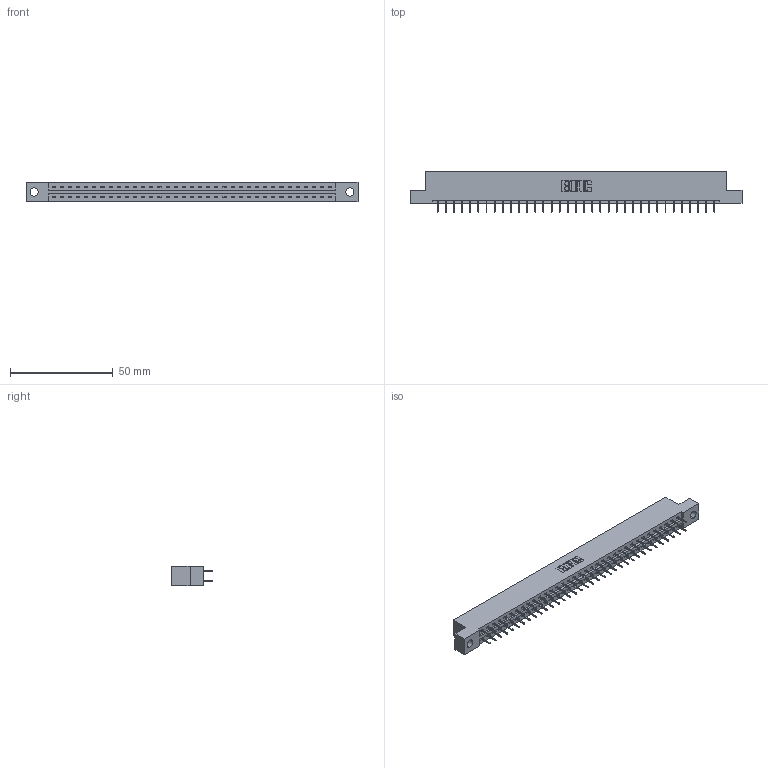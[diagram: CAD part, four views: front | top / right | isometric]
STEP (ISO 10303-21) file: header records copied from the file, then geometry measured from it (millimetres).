
FILE_DESCRIPTION (( 'STEP AP203' ), '1' );
FILE_NAME ('387-070-524-204.STEP', '2019-10-19T23:07:58', ( '' ), ( '' ), 'SwSTEP 2.0', 'SolidWorks 2016', '' );
FILE_SCHEMA (( 'CONFIG_CONTROL_DESIGN' ));
Length unit declared in the file: inch
Products named in the file (3): 387-070-524-204; 337 Part_Flush Mounting Lugs - 0.156 Dia-TH; 345-292-001_345-293-124
Assembly tree (71 placements, depth 2):
  387-070-524-204
    337 Part_Flush Mounting Lugs - 0.156 Dia-TH
    345-292-001_345-293-124  x70
Bounding box: 161.7 x 19.69 x 9.4 mm (x, y, z)
Volume: 16753.9 mm3; surface area: 18341.6 mm2
Topology: 71 solids, 71 shells, 4174 faces, 11861 edges, 7626 vertices
Faces by surface type: plane 3150, cylinder 1024
Entity records: 28119 total; most frequent: CARTESIAN_POINT 4742, ORIENTED_EDGE 4678, DIRECTION 4047, EDGE_CURVE 2339, LINE 2215, VECTOR 2215, VERTEX_POINT 1554, AXIS2_PLACEMENT_3D 916
